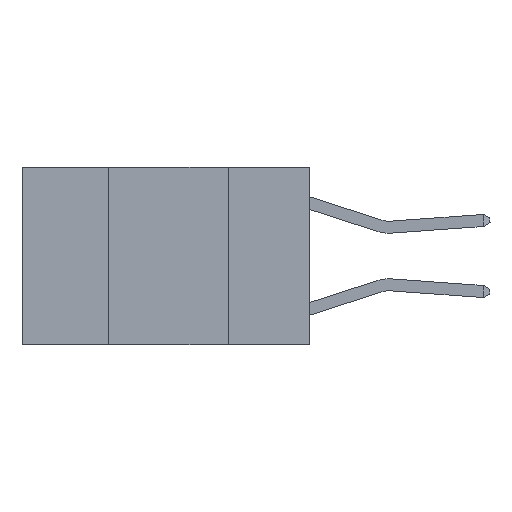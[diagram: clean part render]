
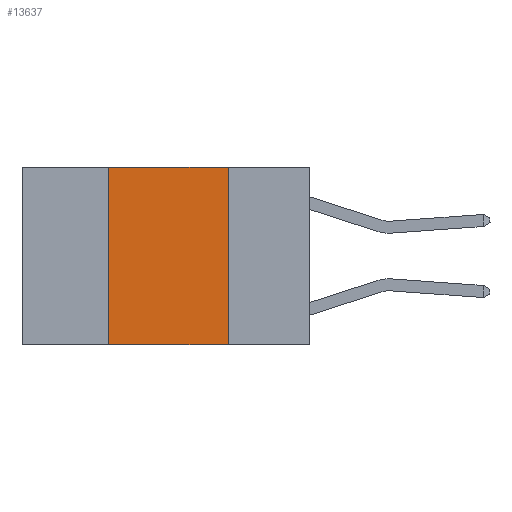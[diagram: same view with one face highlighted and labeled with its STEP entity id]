
A CAD part, left-side view. The second image highlights one B-rep face of the part: STEP entity #13637.
In plain terms, the highlighted planar face has unit normal (-1, 0, 0).
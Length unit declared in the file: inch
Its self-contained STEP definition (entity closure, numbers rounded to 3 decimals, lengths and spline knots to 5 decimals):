
#29 = VECTOR ( 'NONE', #14967, 39.37008 ) ;
#900 = EDGE_CURVE ( 'NONE', #10675, #2205, #8065, .T. ) ;
#979 = DIRECTION ( 'NONE',  ( 0., 0., -1. ) ) ;
#2205 = VERTEX_POINT ( 'NONE', #10371 ) ;
#2689 = EDGE_LOOP ( 'NONE', ( #18201, #13391, #8665, #19002 ) ) ;
#2976 = DIRECTION ( 'NONE',  ( 0., -1., 0. ) ) ;
#4639 = VERTEX_POINT ( 'NONE', #6289 ) ;
#4865 = LINE ( 'NONE', #11907, #8132 ) ;
#5935 = DIRECTION ( 'NONE',  ( 0., 0., 1. ) ) ;
#6289 = CARTESIAN_POINT ( 'NONE',  ( 0., 0.42, 0. ) ) ;
#6997 = CARTESIAN_POINT ( 'NONE',  ( 0., 0.6, 0. ) ) ;
#8065 = LINE ( 'NONE', #13435, #29 ) ;
#8132 = VECTOR ( 'NONE', #5935, 39.37008 ) ;
#8203 = VECTOR ( 'NONE', #10489, 39.37008 ) ;
#8665 = ORIENTED_EDGE ( 'NONE', *, *, #17938, .F. ) ;
#8702 = LINE ( 'NONE', #19467, #8203 ) ;
#9743 = LINE ( 'NONE', #18075, #17264 ) ;
#10030 = DIRECTION ( 'NONE',  ( 1., 0., 0. ) ) ;
#10371 = CARTESIAN_POINT ( 'NONE',  ( 0., 0.17, -0.37 ) ) ;
#10461 = CARTESIAN_POINT ( 'NONE',  ( 0., 0.17, 0. ) ) ;
#10489 = DIRECTION ( 'NONE',  ( 0., 0., -1. ) ) ;
#10675 = VERTEX_POINT ( 'NONE', #16611 ) ;
#11907 = CARTESIAN_POINT ( 'NONE',  ( 0., 0.42, 0. ) ) ;
#11924 = VERTEX_POINT ( 'NONE', #10461 ) ;
#11954 = EDGE_CURVE ( 'NONE', #4639, #11924, #9743, .T. ) ;
#13391 = ORIENTED_EDGE ( 'NONE', *, *, #11954, .F. ) ;
#13435 = CARTESIAN_POINT ( 'NONE',  ( 0., 0.6, -0.37 ) ) ;
#13637 = ADVANCED_FACE ( 'NONE', ( #13711 ), #19010, .F. ) ;
#13711 = FACE_OUTER_BOUND ( 'NONE', #2689, .T. ) ;
#14967 = DIRECTION ( 'NONE',  ( 0., -1., 0. ) ) ;
#15431 = EDGE_CURVE ( 'NONE', #11924, #2205, #8702, .T. ) ;
#16611 = CARTESIAN_POINT ( 'NONE',  ( 0., 0.42, -0.37 ) ) ;
#17264 = VECTOR ( 'NONE', #2976, 39.37008 ) ;
#17938 = EDGE_CURVE ( 'NONE', #10675, #4639, #4865, .T. ) ;
#18075 = CARTESIAN_POINT ( 'NONE',  ( 0., 0.6, 0. ) ) ;
#18201 = ORIENTED_EDGE ( 'NONE', *, *, #15431, .F. ) ;
#18778 = AXIS2_PLACEMENT_3D ( 'NONE', #6997, #10030, #979 ) ;
#19002 = ORIENTED_EDGE ( 'NONE', *, *, #900, .T. ) ;
#19010 = PLANE ( 'NONE',  #18778 ) ;
#19467 = CARTESIAN_POINT ( 'NONE',  ( 0., 0.17, 0. ) ) ;
